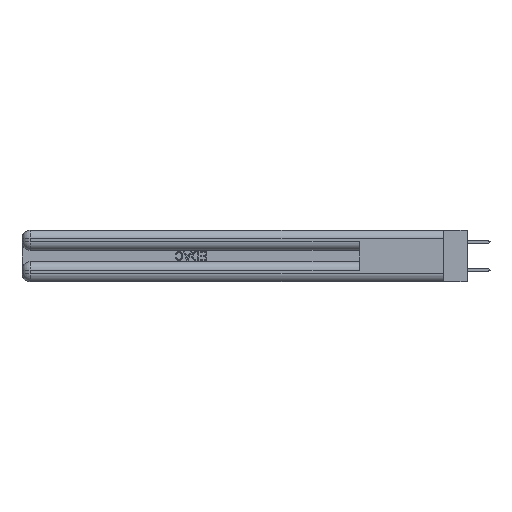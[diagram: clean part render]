
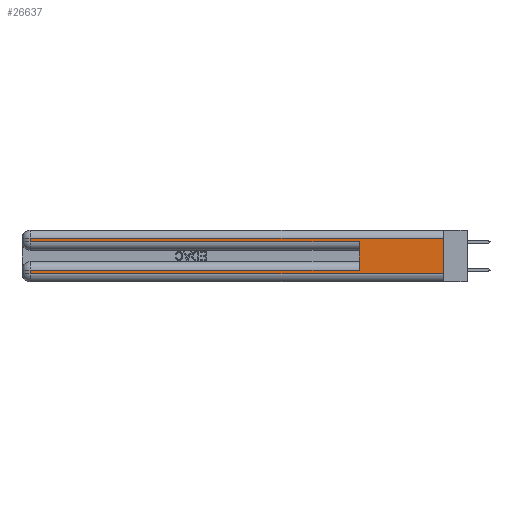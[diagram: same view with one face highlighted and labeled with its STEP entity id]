
A CAD part, left-side view. The second image highlights one B-rep face of the part: STEP entity #26637.
In plain terms, the highlighted planar face has unit normal (-1, 0, 0).
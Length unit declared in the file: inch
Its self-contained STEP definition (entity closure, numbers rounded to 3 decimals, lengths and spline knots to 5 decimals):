
#341 = VECTOR ( 'NONE', #23916, 39.37008 ) ;
#353 = VERTEX_POINT ( 'NONE', #37646 ) ;
#740 = LINE ( 'NONE', #1172, #23237 ) ;
#1110 = VERTEX_POINT ( 'NONE', #10005 ) ;
#1172 = CARTESIAN_POINT ( 'NONE',  ( 0., 0., 0.37 ) ) ;
#1686 = LINE ( 'NONE', #18340, #15991 ) ;
#2061 = EDGE_CURVE ( 'NONE', #16635, #5175, #26568, .T. ) ;
#3377 = DIRECTION ( 'NONE',  ( 0., -1., 0. ) ) ;
#3586 = PLANE ( 'NONE',  #27000 ) ;
#4102 = VERTEX_POINT ( 'NONE', #4652 ) ;
#4652 = CARTESIAN_POINT ( 'NONE',  ( 0., 0., 0.06 ) ) ;
#4912 = VECTOR ( 'NONE', #6634, 39.37008 ) ;
#5175 = VERTEX_POINT ( 'NONE', #20774 ) ;
#5770 = CARTESIAN_POINT ( 'NONE',  ( 0., 0.6, 0.085 ) ) ;
#6607 = DIRECTION ( 'NONE',  ( 1., 0., 0. ) ) ;
#6634 = DIRECTION ( 'NONE',  ( 0., 0., -1. ) ) ;
#7046 = LINE ( 'NONE', #32301, #29326 ) ;
#8306 = LINE ( 'NONE', #18038, #341 ) ;
#8680 = CARTESIAN_POINT ( 'NONE',  ( 0., 2.94, 0.06 ) ) ;
#9556 = LINE ( 'NONE', #29658, #24088 ) ;
#10005 = CARTESIAN_POINT ( 'NONE',  ( 0., 2.94, 0.285 ) ) ;
#10613 = VERTEX_POINT ( 'NONE', #8680 ) ;
#10675 = CARTESIAN_POINT ( 'NONE',  ( 0., 0.6, 0.285 ) ) ;
#12663 = LINE ( 'NONE', #21127, #4912 ) ;
#13704 = CARTESIAN_POINT ( 'NONE',  ( 0., 0., 0.31 ) ) ;
#14092 = CARTESIAN_POINT ( 'NONE',  ( 0., 0.6, 0.145 ) ) ;
#15747 = VERTEX_POINT ( 'NONE', #10675 ) ;
#15871 = EDGE_CURVE ( 'NONE', #16635, #15747, #35584, .T. ) ;
#15991 = VECTOR ( 'NONE', #26882, 39.37008 ) ;
#16635 = VERTEX_POINT ( 'NONE', #5770 ) ;
#17366 = EDGE_CURVE ( 'NONE', #32281, #353, #8306, .T. ) ;
#18038 = CARTESIAN_POINT ( 'NONE',  ( 0., 0., 0.31 ) ) ;
#18340 = CARTESIAN_POINT ( 'NONE',  ( 0., 2.94, 0.37 ) ) ;
#19754 = VECTOR ( 'NONE', #20480, 39.37008 ) ;
#19853 = EDGE_CURVE ( 'NONE', #32281, #4102, #740, .T. ) ;
#20300 = EDGE_CURVE ( 'NONE', #1110, #15747, #9556, .T. ) ;
#20480 = DIRECTION ( 'NONE',  ( 0., 1., 0. ) ) ;
#20774 = CARTESIAN_POINT ( 'NONE',  ( 0., 2.94, 0.085 ) ) ;
#21127 = CARTESIAN_POINT ( 'NONE',  ( 0., 2.94, 0.37 ) ) ;
#22532 = ORIENTED_EDGE ( 'NONE', *, *, #23823, .T. ) ;
#22825 = FACE_OUTER_BOUND ( 'NONE', #25423, .T. ) ;
#23237 = VECTOR ( 'NONE', #36177, 39.37008 ) ;
#23823 = EDGE_CURVE ( 'NONE', #10613, #4102, #7046, .T. ) ;
#23916 = DIRECTION ( 'NONE',  ( 0., 1., 0. ) ) ;
#24006 = CARTESIAN_POINT ( 'NONE',  ( 0., 0., 0.37 ) ) ;
#24088 = VECTOR ( 'NONE', #3377, 39.37008 ) ;
#24656 = ORIENTED_EDGE ( 'NONE', *, *, #2061, .T. ) ;
#25423 = EDGE_LOOP ( 'NONE', ( #29847, #28038, #30965, #32036, #35049, #24656, #37382, #22532 ) ) ;
#26568 = LINE ( 'NONE', #28282, #19754 ) ;
#26637 = ADVANCED_FACE ( 'NONE', ( #22825 ), #3586, .F. ) ;
#26882 = DIRECTION ( 'NONE',  ( 0., 0., -1. ) ) ;
#26928 = DIRECTION ( 'NONE',  ( 0., 0., -1. ) ) ;
#27000 = AXIS2_PLACEMENT_3D ( 'NONE', #24006, #6607, #26928 ) ;
#27050 = VECTOR ( 'NONE', #34338, 39.37008 ) ;
#27359 = EDGE_CURVE ( 'NONE', #353, #1110, #1686, .T. ) ;
#28038 = ORIENTED_EDGE ( 'NONE', *, *, #17366, .T. ) ;
#28282 = CARTESIAN_POINT ( 'NONE',  ( 0., 0., 0.085 ) ) ;
#29326 = VECTOR ( 'NONE', #35178, 39.37008 ) ;
#29658 = CARTESIAN_POINT ( 'NONE',  ( 0., 0., 0.285 ) ) ;
#29847 = ORIENTED_EDGE ( 'NONE', *, *, #19853, .F. ) ;
#30965 = ORIENTED_EDGE ( 'NONE', *, *, #27359, .T. ) ;
#32036 = ORIENTED_EDGE ( 'NONE', *, *, #20300, .T. ) ;
#32062 = EDGE_CURVE ( 'NONE', #5175, #10613, #12663, .T. ) ;
#32281 = VERTEX_POINT ( 'NONE', #13704 ) ;
#32301 = CARTESIAN_POINT ( 'NONE',  ( 0., 0., 0.06 ) ) ;
#34338 = DIRECTION ( 'NONE',  ( 0., 0., 1. ) ) ;
#35049 = ORIENTED_EDGE ( 'NONE', *, *, #15871, .F. ) ;
#35178 = DIRECTION ( 'NONE',  ( 0., -1., 0. ) ) ;
#35584 = LINE ( 'NONE', #14092, #27050 ) ;
#36177 = DIRECTION ( 'NONE',  ( 0., 0., -1. ) ) ;
#37382 = ORIENTED_EDGE ( 'NONE', *, *, #32062, .T. ) ;
#37646 = CARTESIAN_POINT ( 'NONE',  ( 0., 2.94, 0.31 ) ) ;
